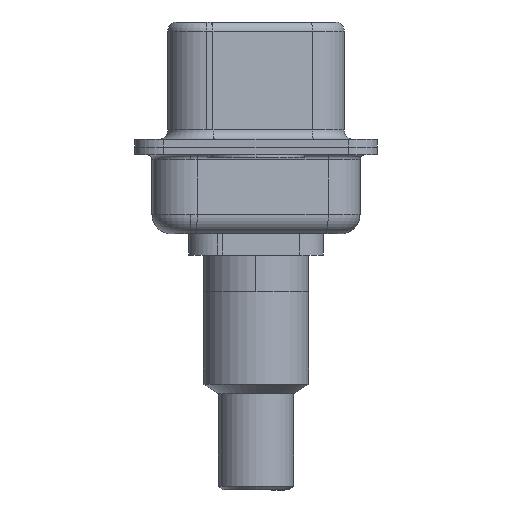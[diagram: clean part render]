
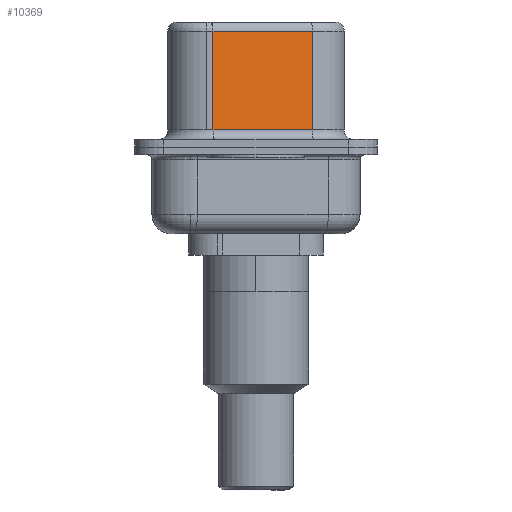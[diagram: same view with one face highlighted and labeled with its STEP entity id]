
A CAD part, left-side view. The second image highlights one B-rep face of the part: STEP entity #10369.
In plain terms, the highlighted planar face has unit normal (-0.985, -0.174, 0).
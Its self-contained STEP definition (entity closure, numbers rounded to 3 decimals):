
#413 = VECTOR ( 'NONE', #13513, 1000. ) ;
#925 = VERTEX_POINT ( 'NONE', #15127 ) ;
#1589 = LINE ( 'NONE', #2096, #413 ) ;
#2096 = CARTESIAN_POINT ( 'NONE',  ( 4.58, -2.927, 6.02 ) ) ;
#4710 = DIRECTION ( 'NONE',  ( -0.174, 0.985, 0. ) ) ;
#5922 = AXIS2_PLACEMENT_3D ( 'NONE', #8461, #16063, #4710 ) ;
#6742 = CARTESIAN_POINT ( 'NONE',  ( 3.67, 2.233, 0.9 ) ) ;
#7726 = ORIENTED_EDGE ( 'NONE', *, *, #15603, .F. ) ;
#8043 = VECTOR ( 'NONE', #14770, 1000. ) ;
#8461 = CARTESIAN_POINT ( 'NONE',  ( 4.58, -2.927, 6.52 ) ) ;
#8711 = CARTESIAN_POINT ( 'NONE',  ( 3.67, 2.233, 6.02 ) ) ;
#9911 = EDGE_CURVE ( 'NONE', #21167, #925, #24515, .T. ) ;
#10369 = ADVANCED_FACE ( 'NONE', ( #19674 ), #23768, .F. ) ;
#10568 = VECTOR ( 'NONE', #15769, 1000. ) ;
#11157 = LINE ( 'NONE', #17688, #10568 ) ;
#12873 = CARTESIAN_POINT ( 'NONE',  ( 4.58, -2.927, 0.9 ) ) ;
#13513 = DIRECTION ( 'NONE',  ( -0.174, 0.985, 0. ) ) ;
#13643 = EDGE_CURVE ( 'NONE', #17318, #21167, #15098, .T. ) ;
#13951 = ORIENTED_EDGE ( 'NONE', *, *, #13643, .T. ) ;
#14338 = ORIENTED_EDGE ( 'NONE', *, *, #9911, .T. ) ;
#14770 = DIRECTION ( 'NONE',  ( 0.174, -0.985, 0. ) ) ;
#14956 = DIRECTION ( 'NONE',  ( 0., 0., -1. ) ) ;
#15098 = LINE ( 'NONE', #18807, #19582 ) ;
#15127 = CARTESIAN_POINT ( 'NONE',  ( 4.58, -2.927, 0.9 ) ) ;
#15603 = EDGE_CURVE ( 'NONE', #19030, #925, #11157, .T. ) ;
#15769 = DIRECTION ( 'NONE',  ( 0., 0., -1. ) ) ;
#16063 = DIRECTION ( 'NONE',  ( 0.985, 0.174, 0. ) ) ;
#16131 = EDGE_CURVE ( 'NONE', #19030, #17318, #1589, .T. ) ;
#17293 = EDGE_LOOP ( 'NONE', ( #7726, #22227, #13951, #14338 ) ) ;
#17318 = VERTEX_POINT ( 'NONE', #8711 ) ;
#17688 = CARTESIAN_POINT ( 'NONE',  ( 4.58, -2.927, 6.52 ) ) ;
#18807 = CARTESIAN_POINT ( 'NONE',  ( 3.67, 2.233, 6.52 ) ) ;
#19030 = VERTEX_POINT ( 'NONE', #23777 ) ;
#19582 = VECTOR ( 'NONE', #14956, 1000. ) ;
#19674 = FACE_OUTER_BOUND ( 'NONE', #17293, .T. ) ;
#21167 = VERTEX_POINT ( 'NONE', #6742 ) ;
#22227 = ORIENTED_EDGE ( 'NONE', *, *, #16131, .T. ) ;
#23768 = PLANE ( 'NONE',  #5922 ) ;
#23777 = CARTESIAN_POINT ( 'NONE',  ( 4.58, -2.927, 6.02 ) ) ;
#24515 = LINE ( 'NONE', #12873, #8043 ) ;
